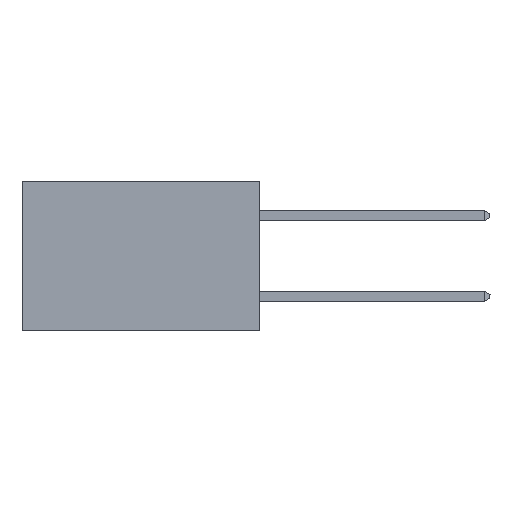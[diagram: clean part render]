
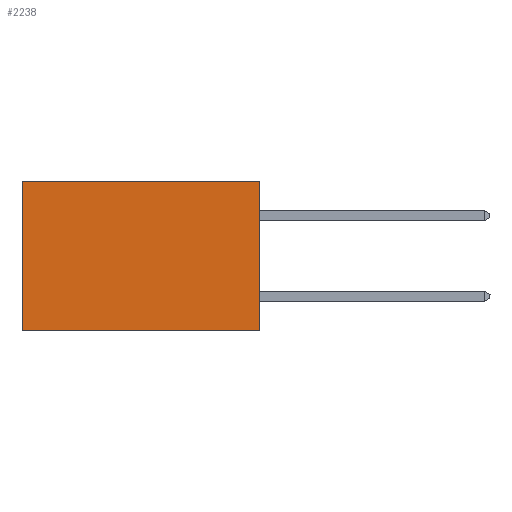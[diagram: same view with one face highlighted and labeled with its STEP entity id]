
A CAD part, left-side view. The second image highlights one B-rep face of the part: STEP entity #2238.
In plain terms, the highlighted planar face has unit normal (-1, 0, 0).
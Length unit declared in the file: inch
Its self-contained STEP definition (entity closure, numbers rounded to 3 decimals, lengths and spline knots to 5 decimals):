
#947 = PLANE ( 'NONE',  #9576 ) ;
#1715 = DIRECTION ( 'NONE',  ( 0., 0., -1. ) ) ;
#2238 = ADVANCED_FACE ( 'NONE', ( #25976 ), #947, .F. ) ;
#2333 = EDGE_CURVE ( 'NONE', #9773, #13993, #9039, .T. ) ;
#2429 = VECTOR ( 'NONE', #13270, 39.37008 ) ;
#5355 = VECTOR ( 'NONE', #7008, 39.37008 ) ;
#5471 = LINE ( 'NONE', #22769, #12875 ) ;
#5824 = CARTESIAN_POINT ( 'NONE',  ( 0.277, 0., -0.37 ) ) ;
#6463 = CARTESIAN_POINT ( 'NONE',  ( 0.277, 0.59, -0.37 ) ) ;
#6544 = VECTOR ( 'NONE', #13455, 39.37008 ) ;
#6881 = CARTESIAN_POINT ( 'NONE',  ( 0.277, 0., 0. ) ) ;
#7008 = DIRECTION ( 'NONE',  ( 0., 0., -1. ) ) ;
#7969 = DIRECTION ( 'NONE',  ( 0., 1., 0. ) ) ;
#9039 = LINE ( 'NONE', #5824, #2429 ) ;
#9576 = AXIS2_PLACEMENT_3D ( 'NONE', #14921, #31514, #1715 ) ;
#9773 = VERTEX_POINT ( 'NONE', #29244 ) ;
#12875 = VECTOR ( 'NONE', #7969, 39.37008 ) ;
#13156 = LINE ( 'NONE', #13345, #6544 ) ;
#13270 = DIRECTION ( 'NONE',  ( 0., 1., 0. ) ) ;
#13345 = CARTESIAN_POINT ( 'NONE',  ( 0.277, 0.59, -0.37 ) ) ;
#13455 = DIRECTION ( 'NONE',  ( 0., 0., -1. ) ) ;
#13993 = VERTEX_POINT ( 'NONE', #6463 ) ;
#14236 = VERTEX_POINT ( 'NONE', #22213 ) ;
#14921 = CARTESIAN_POINT ( 'NONE',  ( 0.277, 0., -0.37 ) ) ;
#15905 = EDGE_LOOP ( 'NONE', ( #19648, #17804, #21457, #22058 ) ) ;
#17007 = EDGE_CURVE ( 'NONE', #25758, #9773, #18507, .T. ) ;
#17804 = ORIENTED_EDGE ( 'NONE', *, *, #2333, .F. ) ;
#18507 = LINE ( 'NONE', #19323, #5355 ) ;
#19323 = CARTESIAN_POINT ( 'NONE',  ( 0.277, 0., -0.37 ) ) ;
#19648 = ORIENTED_EDGE ( 'NONE', *, *, #26905, .T. ) ;
#21457 = ORIENTED_EDGE ( 'NONE', *, *, #17007, .F. ) ;
#22058 = ORIENTED_EDGE ( 'NONE', *, *, #25381, .T. ) ;
#22213 = CARTESIAN_POINT ( 'NONE',  ( 0.277, 0.59, 0. ) ) ;
#22769 = CARTESIAN_POINT ( 'NONE',  ( 0.277, 0., 0. ) ) ;
#25381 = EDGE_CURVE ( 'NONE', #25758, #14236, #5471, .T. ) ;
#25758 = VERTEX_POINT ( 'NONE', #6881 ) ;
#25976 = FACE_OUTER_BOUND ( 'NONE', #15905, .T. ) ;
#26905 = EDGE_CURVE ( 'NONE', #14236, #13993, #13156, .T. ) ;
#29244 = CARTESIAN_POINT ( 'NONE',  ( 0.277, 0., -0.37 ) ) ;
#31514 = DIRECTION ( 'NONE',  ( 1., 0., 0. ) ) ;
